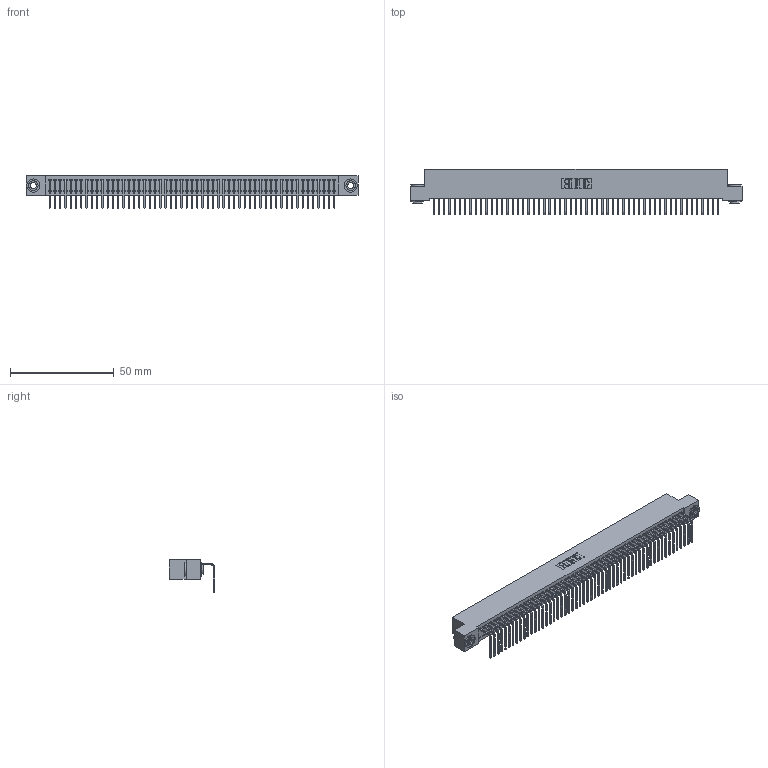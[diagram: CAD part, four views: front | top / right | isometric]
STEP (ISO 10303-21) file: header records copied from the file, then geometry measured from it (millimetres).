
FILE_DESCRIPTION (( 'STEP AP203' ), '1' );
FILE_NAME ('392-055-558-103.STEP', '2018-08-17T11:34:54', ( '' ), ( '' ), 'SwSTEP 2.0', 'SolidWorks 2016', '' );
FILE_SCHEMA (( 'CONFIG_CONTROL_DESIGN' ));
Length unit declared in the file: inch
Products named in the file (4): 342 Part_.156 TH; 345-292-001_558 Tail - 2; 342-250-002_345-250-002-102; 392-055-558-103
Assembly tree (58 placements, depth 2):
  392-055-558-103
    342 Part_.156 TH
    345-292-001_558 Tail - 2  x55
    342-250-002_345-250-002-102  x2
Bounding box: 160.02 x 21.91 x 15.62 mm (x, y, z)
Volume: 14284.5 mm3; surface area: 22485.8 mm2
Topology: 58 solids, 58 shells, 3448 faces, 10385 edges, 6846 vertices
Faces by surface type: plane 2496, cylinder 944, cone 8
Entity records: 32544 total; most frequent: CARTESIAN_POINT 5590, ORIENTED_EDGE 5574, DIRECTION 4723, EDGE_CURVE 2787, VECTOR 2635, LINE 2635, VERTEX_POINT 1854, AXIS2_PLACEMENT_3D 1044
